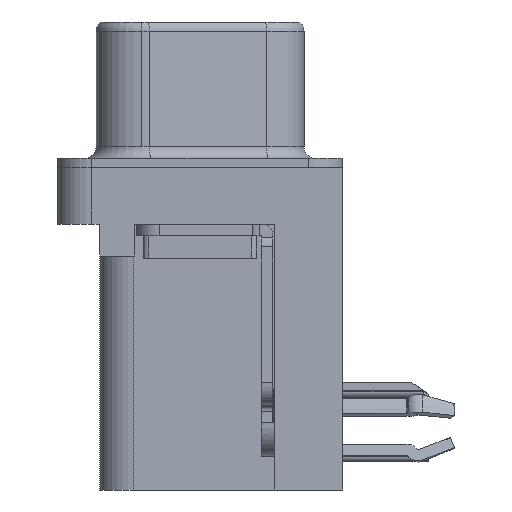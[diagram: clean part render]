
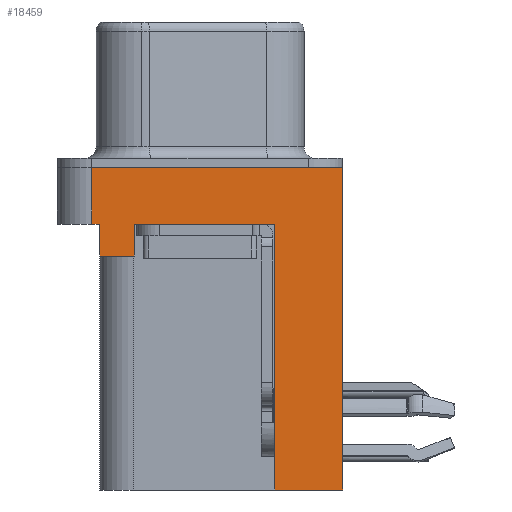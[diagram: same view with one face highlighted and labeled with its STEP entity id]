
A CAD part, left-side view. The second image highlights one B-rep face of the part: STEP entity #18459.
In plain terms, the highlighted planar face has unit normal (-1, 0, 0).
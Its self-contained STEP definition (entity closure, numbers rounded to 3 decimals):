
#70 = CARTESIAN_POINT ( 'NONE',  ( -3., 4.425, -2.5 ) ) ;
#130 = LINE ( 'NONE', #17037, #5637 ) ;
#156 = VECTOR ( 'NONE', #9994, 1000. ) ;
#224 = VECTOR ( 'NONE', #16662, 1000. ) ;
#277 = ORIENTED_EDGE ( 'NONE', *, *, #6637, .F. ) ;
#528 = CARTESIAN_POINT ( 'NONE',  ( -3., 4.775, -2.5 ) ) ;
#653 = VERTEX_POINT ( 'NONE', #23411 ) ;
#1868 = VERTEX_POINT ( 'NONE', #18975 ) ;
#1971 = VERTEX_POINT ( 'NONE', #21181 ) ;
#2561 = DIRECTION ( 'NONE',  ( 0., 0., 1. ) ) ;
#2924 = EDGE_CURVE ( 'NONE', #1971, #1868, #130, .T. ) ;
#2984 = VERTEX_POINT ( 'NONE', #4921 ) ;
#3335 = LINE ( 'NONE', #12839, #224 ) ;
#3405 = DIRECTION ( 'NONE',  ( 0., 0., 1. ) ) ;
#3605 = DIRECTION ( 'NONE',  ( 0., 1., 0. ) ) ;
#3994 = LINE ( 'NONE', #9779, #20482 ) ;
#4246 = ORIENTED_EDGE ( 'NONE', *, *, #14130, .T. ) ;
#4252 = ORIENTED_EDGE ( 'NONE', *, *, #19982, .F. ) ;
#4718 = EDGE_CURVE ( 'NONE', #13565, #2984, #6529, .T. ) ;
#4800 = VERTEX_POINT ( 'NONE', #70 ) ;
#4884 = VECTOR ( 'NONE', #3605, 1000. ) ;
#4888 = DIRECTION ( 'NONE',  ( 0., -1., 0. ) ) ;
#4921 = CARTESIAN_POINT ( 'NONE',  ( -3., -6.275, 0. ) ) ;
#5637 = VECTOR ( 'NONE', #8490, 1000. ) ;
#5833 = VECTOR ( 'NONE', #4888, 1000. ) ;
#6259 = VECTOR ( 'NONE', #21573, 1000. ) ;
#6529 = LINE ( 'NONE', #14047, #6259 ) ;
#6552 = ORIENTED_EDGE ( 'NONE', *, *, #13197, .F. ) ;
#6637 = EDGE_CURVE ( 'NONE', #11722, #24010, #20311, .T. ) ;
#6748 = CARTESIAN_POINT ( 'NONE',  ( -3., 2.895, -2.5 ) ) ;
#7071 = CARTESIAN_POINT ( 'NONE',  ( -3., -3.295, -14.2 ) ) ;
#7166 = CARTESIAN_POINT ( 'NONE',  ( -3., 4.425, -3.9 ) ) ;
#7427 = LINE ( 'NONE', #7071, #4884 ) ;
#7802 = CARTESIAN_POINT ( 'NONE',  ( -3., -3.295, -2.5 ) ) ;
#8236 = VECTOR ( 'NONE', #17929, 1000. ) ;
#8490 = DIRECTION ( 'NONE',  ( 0., 1., 0. ) ) ;
#9464 = ORIENTED_EDGE ( 'NONE', *, *, #2924, .F. ) ;
#9720 = ORIENTED_EDGE ( 'NONE', *, *, #21598, .T. ) ;
#9779 = CARTESIAN_POINT ( 'NONE',  ( -3., -6.275, -2.5 ) ) ;
#9796 = EDGE_CURVE ( 'NONE', #12396, #24010, #23428, .T. ) ;
#9994 = DIRECTION ( 'NONE',  ( 0., 0., 1. ) ) ;
#10125 = CARTESIAN_POINT ( 'NONE',  ( -3., 2.895, -3.9 ) ) ;
#11071 = ORIENTED_EDGE ( 'NONE', *, *, #21797, .T. ) ;
#11517 = DIRECTION ( 'NONE',  ( 0., 0., 1. ) ) ;
#11722 = VERTEX_POINT ( 'NONE', #22269 ) ;
#11744 = LINE ( 'NONE', #10125, #17951 ) ;
#12396 = VERTEX_POINT ( 'NONE', #6748 ) ;
#12839 = CARTESIAN_POINT ( 'NONE',  ( -3., -6.275, -2.5 ) ) ;
#13197 = EDGE_CURVE ( 'NONE', #1868, #4800, #16199, .T. ) ;
#13565 = VERTEX_POINT ( 'NONE', #21835 ) ;
#13605 = DIRECTION ( 'NONE',  ( 0., 0., 1. ) ) ;
#13630 = ORIENTED_EDGE ( 'NONE', *, *, #4718, .F. ) ;
#14047 = CARTESIAN_POINT ( 'NONE',  ( -3., -6.275, 0. ) ) ;
#14130 = EDGE_CURVE ( 'NONE', #653, #2984, #3994, .T. ) ;
#15478 = VERTEX_POINT ( 'NONE', #528 ) ;
#16199 = LINE ( 'NONE', #7166, #8236 ) ;
#16662 = DIRECTION ( 'NONE',  ( 0., -1., 0. ) ) ;
#17037 = CARTESIAN_POINT ( 'NONE',  ( -3., 4.425, -3.9 ) ) ;
#17846 = ORIENTED_EDGE ( 'NONE', *, *, #9796, .T. ) ;
#17847 = FACE_OUTER_BOUND ( 'NONE', #22141, .T. ) ;
#17929 = DIRECTION ( 'NONE',  ( 0., 0., 1. ) ) ;
#17951 = VECTOR ( 'NONE', #13605, 1000. ) ;
#18015 = EDGE_CURVE ( 'NONE', #15478, #13565, #19149, .T. ) ;
#18459 = ADVANCED_FACE ( 'NONE', ( #17847 ), #21296, .T. ) ;
#18975 = CARTESIAN_POINT ( 'NONE',  ( -3., 4.425, -3.9 ) ) ;
#19149 = LINE ( 'NONE', #21118, #156 ) ;
#19448 = CARTESIAN_POINT ( 'NONE',  ( -3., -6.275, -2.5 ) ) ;
#19570 = DIRECTION ( 'NONE',  ( -1., 0., 0. ) ) ;
#19701 = CARTESIAN_POINT ( 'NONE',  ( -3., -6.275, -2.5 ) ) ;
#19862 = AXIS2_PLACEMENT_3D ( 'NONE', #19448, #19570, #2561 ) ;
#19982 = EDGE_CURVE ( 'NONE', #653, #11722, #7427, .T. ) ;
#20311 = LINE ( 'NONE', #22413, #24166 ) ;
#20482 = VECTOR ( 'NONE', #11517, 1000. ) ;
#21118 = CARTESIAN_POINT ( 'NONE',  ( -3., 4.775, -2.5 ) ) ;
#21181 = CARTESIAN_POINT ( 'NONE',  ( -3., 2.895, -3.9 ) ) ;
#21296 = PLANE ( 'NONE',  #19862 ) ;
#21573 = DIRECTION ( 'NONE',  ( 0., -1., 0. ) ) ;
#21598 = EDGE_CURVE ( 'NONE', #1971, #12396, #11744, .T. ) ;
#21797 = EDGE_CURVE ( 'NONE', #15478, #4800, #3335, .T. ) ;
#21835 = CARTESIAN_POINT ( 'NONE',  ( -3., 4.775, 0. ) ) ;
#22141 = EDGE_LOOP ( 'NONE', ( #13630, #24194, #11071, #6552, #9464, #9720, #17846, #277, #4252, #4246 ) ) ;
#22269 = CARTESIAN_POINT ( 'NONE',  ( -3., -3.295, -14.2 ) ) ;
#22413 = CARTESIAN_POINT ( 'NONE',  ( -3., -3.295, -14.2 ) ) ;
#23411 = CARTESIAN_POINT ( 'NONE',  ( -3., -6.275, -14.2 ) ) ;
#23428 = LINE ( 'NONE', #19701, #5833 ) ;
#24010 = VERTEX_POINT ( 'NONE', #7802 ) ;
#24166 = VECTOR ( 'NONE', #3405, 1000. ) ;
#24194 = ORIENTED_EDGE ( 'NONE', *, *, #18015, .F. ) ;
